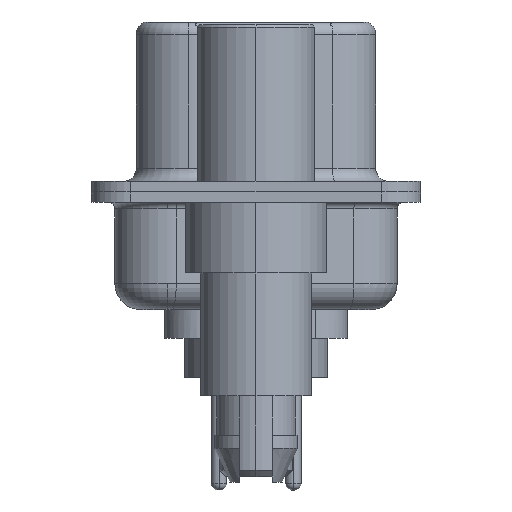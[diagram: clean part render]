
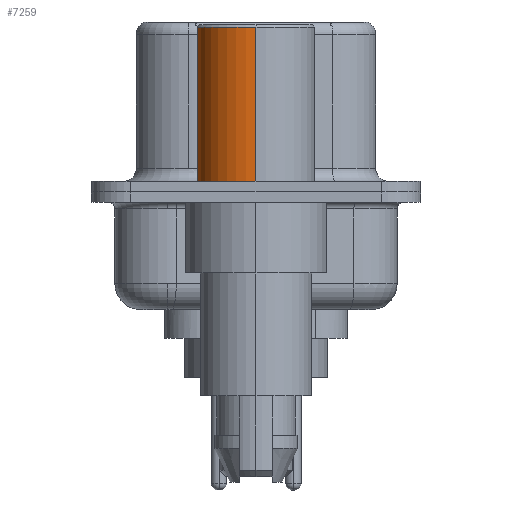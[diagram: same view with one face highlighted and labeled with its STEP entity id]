
A CAD part, left-side view. The second image highlights one B-rep face of the part: STEP entity #7259.
In plain terms, the highlighted cylindrical face has radius 2.25 mm (diameter 4.5 mm), a partial arc.
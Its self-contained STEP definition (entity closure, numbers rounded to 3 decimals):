
#382 = CARTESIAN_POINT ( 'NONE',  ( 0., 0., 0.4 ) ) ;
#2175 = VECTOR ( 'NONE', #14516, 1000. ) ;
#3557 = LINE ( 'NONE', #14865, #14181 ) ;
#3901 = ORIENTED_EDGE ( 'NONE', *, *, #7923, .T. ) ;
#4151 = CARTESIAN_POINT ( 'NONE',  ( -2.25, 0., 0.4 ) ) ;
#5130 = EDGE_CURVE ( 'NONE', #22053, #21151, #3557, .T. ) ;
#5201 = VERTEX_POINT ( 'NONE', #24401 ) ;
#6989 = CARTESIAN_POINT ( 'NONE',  ( 0., 0., 6.3 ) ) ;
#7259 = ADVANCED_FACE ( 'NONE', ( #12376 ), #21745, .T. ) ;
#7923 = EDGE_CURVE ( 'NONE', #14807, #22053, #11758, .T. ) ;
#8965 = DIRECTION ( 'NONE',  ( 1., 0., 0. ) ) ;
#9269 = CARTESIAN_POINT ( 'NONE',  ( 2.25, 0., 0.4 ) ) ;
#10111 = DIRECTION ( 'NONE',  ( 1., 0., 0. ) ) ;
#10381 = AXIS2_PLACEMENT_3D ( 'NONE', #10547, #16493, #19931 ) ;
#10547 = CARTESIAN_POINT ( 'NONE',  ( 0., 0., 0.581 ) ) ;
#11703 = EDGE_CURVE ( 'NONE', #14807, #5201, #22616, .T. ) ;
#11758 = CIRCLE ( 'NONE', #23342, 2.25 ) ;
#12295 = DIRECTION ( 'NONE',  ( 0., 0., 1. ) ) ;
#12376 = FACE_OUTER_BOUND ( 'NONE', #15316, .T. ) ;
#13373 = EDGE_CURVE ( 'NONE', #5201, #21151, #16571, .T. ) ;
#14181 = VECTOR ( 'NONE', #14846, 1000. ) ;
#14516 = DIRECTION ( 'NONE',  ( 0., 0., 1. ) ) ;
#14807 = VERTEX_POINT ( 'NONE', #9269 ) ;
#14846 = DIRECTION ( 'NONE',  ( 0., 0., 1. ) ) ;
#14865 = CARTESIAN_POINT ( 'NONE',  ( -2.25, 0., 0.581 ) ) ;
#15316 = EDGE_LOOP ( 'NONE', ( #3901, #21069, #18317, #16020 ) ) ;
#16020 = ORIENTED_EDGE ( 'NONE', *, *, #11703, .F. ) ;
#16493 = DIRECTION ( 'NONE',  ( 0., 0., 1. ) ) ;
#16571 = CIRCLE ( 'NONE', #17595, 2.25 ) ;
#17595 = AXIS2_PLACEMENT_3D ( 'NONE', #6989, #20273, #8965 ) ;
#18317 = ORIENTED_EDGE ( 'NONE', *, *, #13373, .F. ) ;
#19931 = DIRECTION ( 'NONE',  ( 1., 0., 0. ) ) ;
#20273 = DIRECTION ( 'NONE',  ( 0., 0., 1. ) ) ;
#21069 = ORIENTED_EDGE ( 'NONE', *, *, #5130, .T. ) ;
#21151 = VERTEX_POINT ( 'NONE', #23993 ) ;
#21745 = CYLINDRICAL_SURFACE ( 'NONE', #10381, 2.25 ) ;
#22053 = VERTEX_POINT ( 'NONE', #4151 ) ;
#22616 = LINE ( 'NONE', #23889, #2175 ) ;
#23342 = AXIS2_PLACEMENT_3D ( 'NONE', #382, #12295, #10111 ) ;
#23889 = CARTESIAN_POINT ( 'NONE',  ( 2.25, 0., 0.581 ) ) ;
#23993 = CARTESIAN_POINT ( 'NONE',  ( -2.25, 0., 6.3 ) ) ;
#24401 = CARTESIAN_POINT ( 'NONE',  ( 2.25, 0., 6.3 ) ) ;
